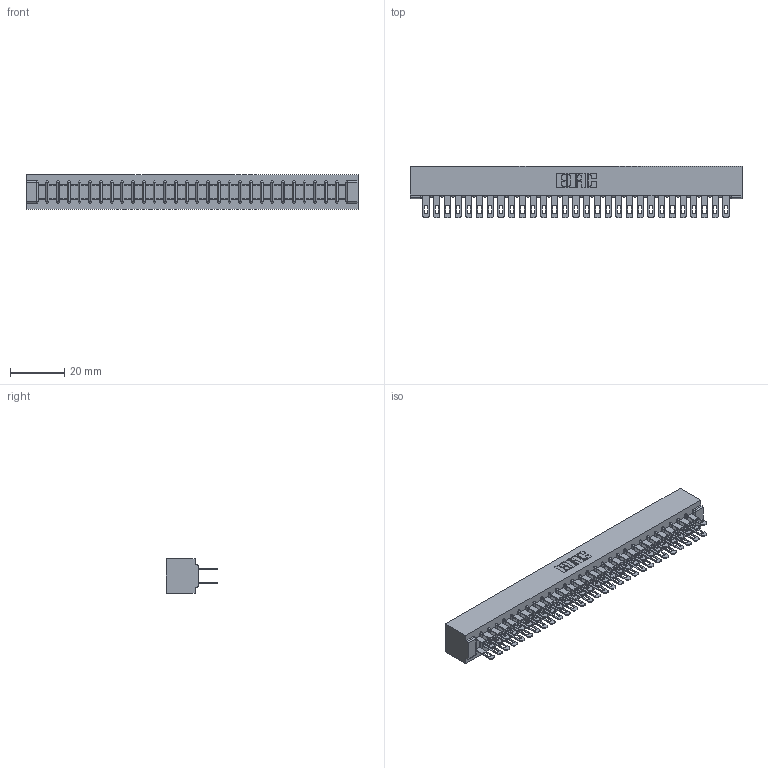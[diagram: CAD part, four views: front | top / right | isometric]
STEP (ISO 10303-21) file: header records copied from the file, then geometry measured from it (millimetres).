
FILE_DESCRIPTION (( 'STEP AP203' ), '1' );
FILE_NAME ('357-058-400-201.STEP', '2020-10-04T11:11:39', ( '' ), ( '' ), 'SwSTEP 2.0', 'SolidWorks 2020', '' );
FILE_SCHEMA (( 'CONFIG_CONTROL_DESIGN' ));
Length unit declared in the file: inch
Products named in the file (3): 357-058-400-201; 307 Part_No Mounting Lugs; 307-290-001_500
Assembly tree (59 placements, depth 2):
  357-058-400-201
    307 Part_No Mounting Lugs
    307-290-001_500  x58
Bounding box: 122.78 x 19.18 x 12.7 mm (x, y, z)
Volume: 13678.2 mm3; surface area: 17711.6 mm2
Topology: 59 solids, 59 shells, 2808 faces, 7839 edges, 5066 vertices
Faces by surface type: plane 1806, cylinder 942, sphere 60
Entity records: 27088 total; most frequent: CARTESIAN_POINT 4429, ORIENTED_EDGE 4386, DIRECTION 4345, EDGE_CURVE 2193, LINE 1677, VECTOR 1677, VERTEX_POINT 1418, AXIS2_PLACEMENT_3D 1334
